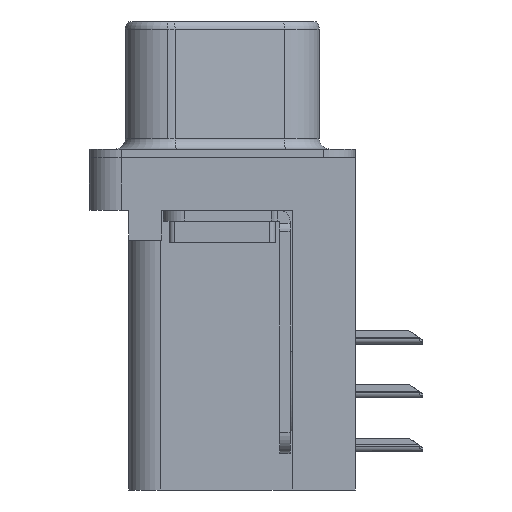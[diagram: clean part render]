
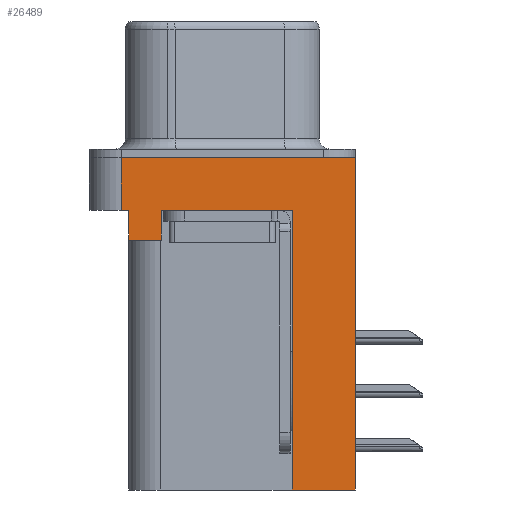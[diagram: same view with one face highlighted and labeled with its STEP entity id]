
A CAD part, left-side view. The second image highlights one B-rep face of the part: STEP entity #26489.
In plain terms, the highlighted planar face has unit normal (-1, 0, 0).
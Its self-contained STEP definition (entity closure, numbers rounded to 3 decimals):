
#503 = VECTOR ( 'NONE', #7285, 1000. ) ;
#594 = LINE ( 'NONE', #14425, #503 ) ;
#696 = VECTOR ( 'NONE', #11971, 1000. ) ;
#770 = VECTOR ( 'NONE', #21079, 1000. ) ;
#794 = LINE ( 'NONE', #9570, #696 ) ;
#829 = LINE ( 'NONE', #18811, #770 ) ;
#887 = VERTEX_POINT ( 'NONE', #9970 ) ;
#952 = VECTOR ( 'NONE', #23368, 1000. ) ;
#1087 = LINE ( 'NONE', #14116, #952 ) ;
#1797 = VECTOR ( 'NONE', #15926, 1000. ) ;
#1958 = LINE ( 'NONE', #27500, #1797 ) ;
#2466 = CARTESIAN_POINT ( 'NONE',  ( -3., -6.275, -2.5 ) ) ;
#2879 = VERTEX_POINT ( 'NONE', #10939 ) ;
#3324 = EDGE_LOOP ( 'NONE', ( #10360, #15804, #15768, #29306, #30280, #22534, #30980, #19824, #30795, #19141 ) ) ;
#3537 = CARTESIAN_POINT ( 'NONE',  ( -3., -3.295, -15.7 ) ) ;
#3547 = CARTESIAN_POINT ( 'NONE',  ( -3., 4.775, -2.5 ) ) ;
#3600 = VERTEX_POINT ( 'NONE', #28576 ) ;
#3903 = VECTOR ( 'NONE', #11329, 1000. ) ;
#4078 = AXIS2_PLACEMENT_3D ( 'NONE', #2466, #5263, #21656 ) ;
#4563 = LINE ( 'NONE', #27540, #3903 ) ;
#5263 = DIRECTION ( 'NONE',  ( -1., 0., 0. ) ) ;
#7108 = CARTESIAN_POINT ( 'NONE',  ( -3., 4.425, -2.5 ) ) ;
#7285 = DIRECTION ( 'NONE',  ( 0., 0., 1. ) ) ;
#7359 = CARTESIAN_POINT ( 'NONE',  ( -3., -3.295, -2.5 ) ) ;
#8306 = CARTESIAN_POINT ( 'NONE',  ( -3., 2.895, -3.9 ) ) ;
#9570 = CARTESIAN_POINT ( 'NONE',  ( -3., -6.275, -2.5 ) ) ;
#9970 = CARTESIAN_POINT ( 'NONE',  ( -3., 2.895, -2.5 ) ) ;
#10113 = DIRECTION ( 'NONE',  ( 0., -1., 0. ) ) ;
#10118 = VECTOR ( 'NONE', #30971, 1000. ) ;
#10360 = ORIENTED_EDGE ( 'NONE', *, *, #17685, .F. ) ;
#10771 = LINE ( 'NONE', #28479, #10118 ) ;
#10939 = CARTESIAN_POINT ( 'NONE',  ( -3., 4.425, -3.9 ) ) ;
#11329 = DIRECTION ( 'NONE',  ( 0., -1., 0. ) ) ;
#11971 = DIRECTION ( 'NONE',  ( 0., 0., 1. ) ) ;
#12125 = CARTESIAN_POINT ( 'NONE',  ( -3., 4.775, 0. ) ) ;
#13166 = CARTESIAN_POINT ( 'NONE',  ( -3., -6.275, -2.5 ) ) ;
#14116 = CARTESIAN_POINT ( 'NONE',  ( -3., -3.295, -15.7 ) ) ;
#14425 = CARTESIAN_POINT ( 'NONE',  ( -3., 4.425, -3.9 ) ) ;
#15687 = CARTESIAN_POINT ( 'NONE',  ( -3., 4.425, -3.9 ) ) ;
#15768 = ORIENTED_EDGE ( 'NONE', *, *, #17893, .T. ) ;
#15804 = ORIENTED_EDGE ( 'NONE', *, *, #17319, .F. ) ;
#15926 = DIRECTION ( 'NONE',  ( 0., 0., 1. ) ) ;
#17193 = VERTEX_POINT ( 'NONE', #3537 ) ;
#17319 = EDGE_CURVE ( 'NONE', #28567, #22841, #1958, .T. ) ;
#17474 = EDGE_CURVE ( 'NONE', #17193, #28914, #1087, .T. ) ;
#17509 = EDGE_CURVE ( 'NONE', #22037, #17193, #829, .T. ) ;
#17514 = EDGE_CURVE ( 'NONE', #22037, #3600, #794, .T. ) ;
#17550 = EDGE_CURVE ( 'NONE', #2879, #23217, #594, .T. ) ;
#17594 = CARTESIAN_POINT ( 'NONE',  ( -3., -6.275, -15.7 ) ) ;
#17685 = EDGE_CURVE ( 'NONE', #22841, #3600, #30432, .T. ) ;
#17893 = EDGE_CURVE ( 'NONE', #28567, #23217, #23548, .T. ) ;
#17983 = EDGE_CURVE ( 'NONE', #24082, #2879, #21325, .T. ) ;
#18336 = EDGE_CURVE ( 'NONE', #24082, #887, #10771, .T. ) ;
#18610 = EDGE_CURVE ( 'NONE', #887, #28914, #4563, .T. ) ;
#18811 = CARTESIAN_POINT ( 'NONE',  ( -3., -3.295, -15.7 ) ) ;
#19141 = ORIENTED_EDGE ( 'NONE', *, *, #17514, .T. ) ;
#19824 = ORIENTED_EDGE ( 'NONE', *, *, #17474, .F. ) ;
#20372 = VECTOR ( 'NONE', #27358, 1000. ) ;
#21079 = DIRECTION ( 'NONE',  ( 0., 1., 0. ) ) ;
#21325 = LINE ( 'NONE', #15687, #20372 ) ;
#21656 = DIRECTION ( 'NONE',  ( 0., 0., 1. ) ) ;
#22037 = VERTEX_POINT ( 'NONE', #17594 ) ;
#22325 = FACE_OUTER_BOUND ( 'NONE', #3324, .T. ) ;
#22534 = ORIENTED_EDGE ( 'NONE', *, *, #18336, .T. ) ;
#22841 = VERTEX_POINT ( 'NONE', #12125 ) ;
#23217 = VERTEX_POINT ( 'NONE', #7108 ) ;
#23368 = DIRECTION ( 'NONE',  ( 0., 0., 1. ) ) ;
#23548 = LINE ( 'NONE', #13166, #24780 ) ;
#24082 = VERTEX_POINT ( 'NONE', #8306 ) ;
#24780 = VECTOR ( 'NONE', #29427, 1000. ) ;
#26363 = CARTESIAN_POINT ( 'NONE',  ( -3., -6.275, 0. ) ) ;
#26489 = ADVANCED_FACE ( 'NONE', ( #22325 ), #31021, .T. ) ;
#27358 = DIRECTION ( 'NONE',  ( 0., 1., 0. ) ) ;
#27500 = CARTESIAN_POINT ( 'NONE',  ( -3., 4.775, -2.5 ) ) ;
#27540 = CARTESIAN_POINT ( 'NONE',  ( -3., -6.275, -2.5 ) ) ;
#28479 = CARTESIAN_POINT ( 'NONE',  ( -3., 2.895, -3.9 ) ) ;
#28567 = VERTEX_POINT ( 'NONE', #3547 ) ;
#28576 = CARTESIAN_POINT ( 'NONE',  ( -3., -6.275, 0. ) ) ;
#28914 = VERTEX_POINT ( 'NONE', #7359 ) ;
#29306 = ORIENTED_EDGE ( 'NONE', *, *, #17550, .F. ) ;
#29427 = DIRECTION ( 'NONE',  ( 0., -1., 0. ) ) ;
#30280 = ORIENTED_EDGE ( 'NONE', *, *, #17983, .F. ) ;
#30363 = VECTOR ( 'NONE', #10113, 1000. ) ;
#30432 = LINE ( 'NONE', #26363, #30363 ) ;
#30795 = ORIENTED_EDGE ( 'NONE', *, *, #17509, .F. ) ;
#30971 = DIRECTION ( 'NONE',  ( 0., 0., 1. ) ) ;
#30980 = ORIENTED_EDGE ( 'NONE', *, *, #18610, .T. ) ;
#31021 = PLANE ( 'NONE',  #4078 ) ;
